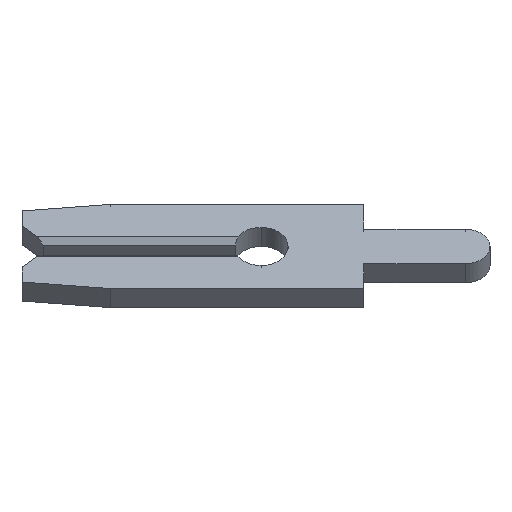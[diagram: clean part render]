
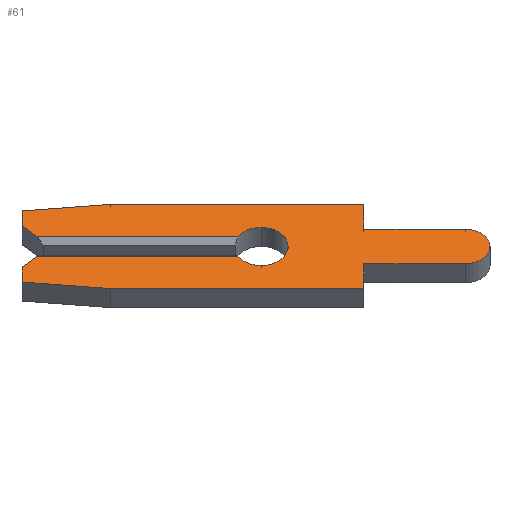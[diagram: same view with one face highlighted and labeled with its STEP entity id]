
A CAD part, left-side view. The second image highlights one B-rep face of the part: STEP entity #61.
In plain terms, the highlighted face is planar.
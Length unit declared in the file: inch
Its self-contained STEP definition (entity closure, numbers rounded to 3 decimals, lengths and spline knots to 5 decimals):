
#1 = CARTESIAN_POINT ( 'NONE',  ( -0.013, 0.216, 0.013 ) ) ;
#2 = VECTOR ( 'NONE', #400, 39.37008 ) ;
#10 = CARTESIAN_POINT ( 'NONE',  ( -0.013, 0.146, -0.0575 ) ) ;
#12 = DIRECTION ( 'NONE',  ( 1., 0., 0. ) ) ;
#14 = LINE ( 'NONE', #392, #177 ) ;
#28 = VECTOR ( 'NONE', #991, 39.37008 ) ;
#50 = ORIENTED_EDGE ( 'NONE', *, *, #1153, .F. ) ;
#53 = DIRECTION ( 'NONE',  ( 0., 0., 1. ) ) ;
#61 = ADVANCED_FACE ( 'NONE', ( #984 ), #391, .F. ) ;
#62 = VECTOR ( 'NONE', #1049, 39.37008 ) ;
#69 = ORIENTED_EDGE ( 'NONE', *, *, #640, .F. ) ;
#72 = AXIS2_PLACEMENT_3D ( 'NONE', #237, #418, #678 ) ;
#74 = VERTEX_POINT ( 'NONE', #598 ) ;
#90 = DIRECTION ( 'NONE',  ( 0., 1., 0. ) ) ;
#93 = DIRECTION ( 'NONE',  ( 0., 0., -1. ) ) ;
#97 = DIRECTION ( 'NONE',  ( -1., 0., 0. ) ) ;
#110 = CARTESIAN_POINT ( 'NONE',  ( -0.013, 0.02252, -0.013 ) ) ;
#111 = VECTOR ( 'NONE', #1086, 39.37008 ) ;
#113 = VECTOR ( 'NONE', #837, 39.37008 ) ;
#114 = ORIENTED_EDGE ( 'NONE', *, *, #726, .F. ) ;
#115 = LINE ( 'NONE', #1060, #510 ) ;
#117 = EDGE_CURVE ( 'NONE', #74, #631, #994, .T. ) ;
#120 = DIRECTION ( 'NONE',  ( 0., 0., -1. ) ) ;
#123 = CARTESIAN_POINT ( 'NONE',  ( -0.013, 0.146, 0.0575 ) ) ;
#124 = EDGE_CURVE ( 'NONE', #892, #760, #154, .T. ) ;
#137 = CIRCLE ( 'NONE', #430, 0.026 ) ;
#139 = ORIENTED_EDGE ( 'NONE', *, *, #152, .F. ) ;
#152 = EDGE_CURVE ( 'NONE', #240, #325, #115, .T. ) ;
#154 = CIRCLE ( 'NONE', #72, 0.026 ) ;
#157 = ORIENTED_EDGE ( 'NONE', *, *, #511, .F. ) ;
#161 = ORIENTED_EDGE ( 'NONE', *, *, #974, .F. ) ;
#168 = VERTEX_POINT ( 'NONE', #873 ) ;
#177 = VECTOR ( 'NONE', #53, 39.37008 ) ;
#180 = ORIENTED_EDGE ( 'NONE', *, *, #965, .F. ) ;
#182 = EDGE_CURVE ( 'NONE', #325, #973, #843, .T. ) ;
#184 = ORIENTED_EDGE ( 'NONE', *, *, #538, .F. ) ;
#194 = ORIENTED_EDGE ( 'NONE', *, *, #295, .T. ) ;
#200 = DIRECTION ( 'NONE',  ( -1., 0., 0. ) ) ;
#237 = CARTESIAN_POINT ( 'NONE',  ( -0.013, 0., 0. ) ) ;
#240 = VERTEX_POINT ( 'NONE', #245 ) ;
#245 = CARTESIAN_POINT ( 'NONE',  ( -0.013, 0.146, -0.0575 ) ) ;
#246 = CARTESIAN_POINT ( 'NONE',  ( -0.013, -0.099, 0.0235 ) ) ;
#257 = VECTOR ( 'NONE', #449, 39.37008 ) ;
#259 = CARTESIAN_POINT ( 'NONE',  ( -0.013, -0.099, -0.0235 ) ) ;
#261 = VERTEX_POINT ( 'NONE', #246 ) ;
#273 = CARTESIAN_POINT ( 'NONE',  ( -0.013, 0.2105, -0.0075 ) ) ;
#284 = LINE ( 'NONE', #433, #394 ) ;
#286 = LINE ( 'NONE', #659, #62 ) ;
#295 = EDGE_CURVE ( 'NONE', #1118, #524, #945, .T. ) ;
#309 = CARTESIAN_POINT ( 'NONE',  ( -0.013, -0.099, -0.0235 ) ) ;
#310 = CARTESIAN_POINT ( 'NONE',  ( -0.013, 0., -0.013 ) ) ;
#315 = CIRCLE ( 'NONE', #903, 0.026 ) ;
#321 = CARTESIAN_POINT ( 'NONE',  ( -0.013, 0.231, -0.028 ) ) ;
#325 = VERTEX_POINT ( 'NONE', #911 ) ;
#341 = LINE ( 'NONE', #259, #28 ) ;
#347 = VERTEX_POINT ( 'NONE', #722 ) ;
#355 = EDGE_CURVE ( 'NONE', #168, #240, #1066, .T. ) ;
#391 = PLANE ( 'NONE',  #480 ) ;
#392 = CARTESIAN_POINT ( 'NONE',  ( -0.013, 0.231, 0.028 ) ) ;
#394 = VECTOR ( 'NONE', #737, 39.37008 ) ;
#400 = DIRECTION ( 'NONE',  ( 0., 0., 1. ) ) ;
#418 = DIRECTION ( 'NONE',  ( -1., 0., 0. ) ) ;
#430 = AXIS2_PLACEMENT_3D ( 'NONE', #927, #97, #93 ) ;
#432 = CARTESIAN_POINT ( 'NONE',  ( -0.013, -0.1975, 0.0235 ) ) ;
#433 = CARTESIAN_POINT ( 'NONE',  ( -0.013, -0.099, -0.0575 ) ) ;
#449 = DIRECTION ( 'NONE',  ( 0., 0.707, 0.707 ) ) ;
#459 = EDGE_CURVE ( 'NONE', #920, #917, #715, .T. ) ;
#478 = EDGE_CURVE ( 'NONE', #760, #524, #137, .T. ) ;
#480 = AXIS2_PLACEMENT_3D ( 'NONE', #859, #579, #486 ) ;
#482 = CARTESIAN_POINT ( 'NONE',  ( -0.013, 0.231, 0.04857 ) ) ;
#485 = VECTOR ( 'NONE', #822, 39.37008 ) ;
#486 = DIRECTION ( 'NONE',  ( 0., 0., -1. ) ) ;
#496 = CARTESIAN_POINT ( 'NONE',  ( -0.013, 0., -0.026 ) ) ;
#510 = VECTOR ( 'NONE', #583, 39.37008 ) ;
#511 = EDGE_CURVE ( 'NONE', #557, #347, #930, .T. ) ;
#524 = VERTEX_POINT ( 'NONE', #934 ) ;
#529 = CARTESIAN_POINT ( 'NONE',  ( -0.013, 0.2105, 0.0075 ) ) ;
#538 = EDGE_CURVE ( 'NONE', #704, #557, #969, .T. ) ;
#541 = VECTOR ( 'NONE', #596, 39.37008 ) ;
#546 = ORIENTED_EDGE ( 'NONE', *, *, #355, .F. ) ;
#557 = VERTEX_POINT ( 'NONE', #123 ) ;
#561 = DIRECTION ( 'NONE',  ( 0., -0.995, 0.105 ) ) ;
#571 = VECTOR ( 'NONE', #90, 39.37008 ) ;
#579 = DIRECTION ( 'NONE',  ( 1., 0., 0. ) ) ;
#583 = DIRECTION ( 'NONE',  ( 0., 0.995, 0.105 ) ) ;
#588 = VECTOR ( 'NONE', #561, 39.37008 ) ;
#596 = DIRECTION ( 'NONE',  ( 0., -1., 0. ) ) ;
#598 = CARTESIAN_POINT ( 'NONE',  ( -0.013, 0.216, -0.013 ) ) ;
#631 = VERTEX_POINT ( 'NONE', #110 ) ;
#638 = DIRECTION ( 'NONE',  ( 0., 0., 1. ) ) ;
#640 = EDGE_CURVE ( 'NONE', #631, #892, #315, .T. ) ;
#659 = CARTESIAN_POINT ( 'NONE',  ( -0.013, -0.099, 0.0575 ) ) ;
#678 = DIRECTION ( 'NONE',  ( 0., 0., -1. ) ) ;
#704 = VERTEX_POINT ( 'NONE', #482 ) ;
#715 = CIRCLE ( 'NONE', #721, 0.0235 ) ;
#716 = ORIENTED_EDGE ( 'NONE', *, *, #1062, .F. ) ;
#719 = ORIENTED_EDGE ( 'NONE', *, *, #124, .F. ) ;
#721 = AXIS2_PLACEMENT_3D ( 'NONE', #924, #12, #638 ) ;
#722 = CARTESIAN_POINT ( 'NONE',  ( -0.013, -0.099, 0.0575 ) ) ;
#726 = EDGE_CURVE ( 'NONE', #347, #261, #286, .T. ) ;
#737 = DIRECTION ( 'NONE',  ( 0., 0., -1. ) ) ;
#739 = CARTESIAN_POINT ( 'NONE',  ( -0.013, 0.146, 0.0575 ) ) ;
#760 = VERTEX_POINT ( 'NONE', #862 ) ;
#805 = DIRECTION ( 'NONE',  ( 0., -1., 0. ) ) ;
#822 = DIRECTION ( 'NONE',  ( 0., -1., 0. ) ) ;
#833 = EDGE_CURVE ( 'NONE', #919, #704, #14, .T. ) ;
#837 = DIRECTION ( 'NONE',  ( 0., -1., 0. ) ) ;
#843 = LINE ( 'NONE', #321, #2 ) ;
#859 = CARTESIAN_POINT ( 'NONE',  ( -0.013, 0., 0. ) ) ;
#862 = CARTESIAN_POINT ( 'NONE',  ( -0.013, 0., 0.026 ) ) ;
#867 = VERTEX_POINT ( 'NONE', #309 ) ;
#873 = CARTESIAN_POINT ( 'NONE',  ( -0.013, -0.099, -0.0575 ) ) ;
#892 = VERTEX_POINT ( 'NONE', #496 ) ;
#901 = LINE ( 'NONE', #529, #257 ) ;
#903 = AXIS2_PLACEMENT_3D ( 'NONE', #1109, #200, #120 ) ;
#911 = CARTESIAN_POINT ( 'NONE',  ( -0.013, 0.231, -0.04857 ) ) ;
#917 = VERTEX_POINT ( 'NONE', #1139 ) ;
#919 = VERTEX_POINT ( 'NONE', #1073 ) ;
#920 = VERTEX_POINT ( 'NONE', #432 ) ;
#924 = CARTESIAN_POINT ( 'NONE',  ( -0.013, -0.1975, 0. ) ) ;
#927 = CARTESIAN_POINT ( 'NONE',  ( -0.013, 0., 0. ) ) ;
#928 = LINE ( 'NONE', #273, #111 ) ;
#930 = LINE ( 'NONE', #739, #113 ) ;
#934 = CARTESIAN_POINT ( 'NONE',  ( -0.013, 0.02252, 0.013 ) ) ;
#945 = LINE ( 'NONE', #1154, #485 ) ;
#965 = EDGE_CURVE ( 'NONE', #261, #920, #1075, .T. ) ;
#969 = LINE ( 'NONE', #1101, #588 ) ;
#973 = VERTEX_POINT ( 'NONE', #1080 ) ;
#974 = EDGE_CURVE ( 'NONE', #917, #867, #341, .T. ) ;
#982 = VECTOR ( 'NONE', #805, 39.37008 ) ;
#984 = FACE_OUTER_BOUND ( 'NONE', #1024, .T. ) ;
#991 = DIRECTION ( 'NONE',  ( 0., 1., 0. ) ) ;
#994 = LINE ( 'NONE', #310, #541 ) ;
#1013 = ORIENTED_EDGE ( 'NONE', *, *, #478, .F. ) ;
#1018 = ORIENTED_EDGE ( 'NONE', *, *, #117, .F. ) ;
#1024 = EDGE_LOOP ( 'NONE', ( #194, #1013, #719, #69, #1018, #1161, #1106, #139, #546, #716, #161, #1122, #180, #114, #157, #184, #1034, #50 ) ) ;
#1034 = ORIENTED_EDGE ( 'NONE', *, *, #833, .F. ) ;
#1049 = DIRECTION ( 'NONE',  ( 0., 0., -1. ) ) ;
#1060 = CARTESIAN_POINT ( 'NONE',  ( -0.013, 0.231, -0.04857 ) ) ;
#1062 = EDGE_CURVE ( 'NONE', #867, #168, #284, .T. ) ;
#1066 = LINE ( 'NONE', #10, #571 ) ;
#1071 = CARTESIAN_POINT ( 'NONE',  ( -0.013, -0.099, 0.0235 ) ) ;
#1073 = CARTESIAN_POINT ( 'NONE',  ( -0.013, 0.231, 0.028 ) ) ;
#1075 = LINE ( 'NONE', #1071, #982 ) ;
#1080 = CARTESIAN_POINT ( 'NONE',  ( -0.013, 0.231, -0.028 ) ) ;
#1086 = DIRECTION ( 'NONE',  ( 0., -0.707, 0.707 ) ) ;
#1096 = EDGE_CURVE ( 'NONE', #973, #74, #928, .T. ) ;
#1101 = CARTESIAN_POINT ( 'NONE',  ( -0.013, 0.231, 0.04857 ) ) ;
#1106 = ORIENTED_EDGE ( 'NONE', *, *, #182, .F. ) ;
#1109 = CARTESIAN_POINT ( 'NONE',  ( -0.013, 0., 0. ) ) ;
#1118 = VERTEX_POINT ( 'NONE', #1 ) ;
#1122 = ORIENTED_EDGE ( 'NONE', *, *, #459, .F. ) ;
#1139 = CARTESIAN_POINT ( 'NONE',  ( -0.013, -0.1975, -0.0235 ) ) ;
#1153 = EDGE_CURVE ( 'NONE', #1118, #919, #901, .T. ) ;
#1154 = CARTESIAN_POINT ( 'NONE',  ( -0.013, 0.231, 0.013 ) ) ;
#1161 = ORIENTED_EDGE ( 'NONE', *, *, #1096, .F. ) ;
